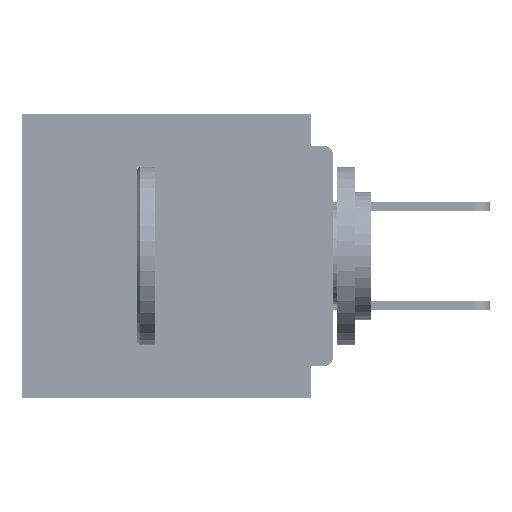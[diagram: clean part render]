
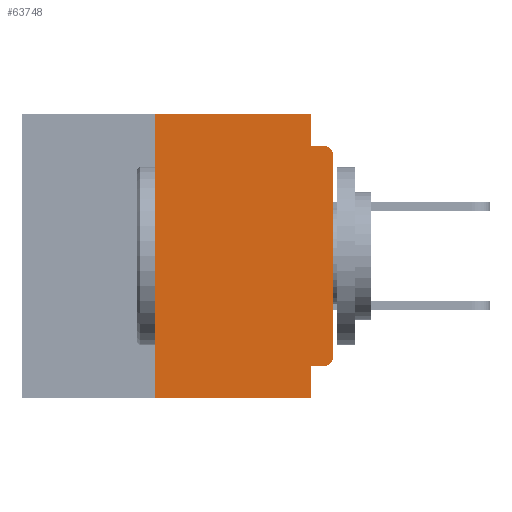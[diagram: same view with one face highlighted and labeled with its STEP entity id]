
A CAD part, left-side view. The second image highlights one B-rep face of the part: STEP entity #63748.
In plain terms, the highlighted planar face has unit normal (-1, 0, 0).
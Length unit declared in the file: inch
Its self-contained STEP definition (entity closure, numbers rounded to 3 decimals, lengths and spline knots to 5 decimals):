
#318 = VECTOR ( 'NONE', #19293, 39.37008 ) ;
#373 = AXIS2_PLACEMENT_3D ( 'NONE', #6621, #44049, #12014 ) ;
#502 = DIRECTION ( 'NONE',  ( 0., 0., -1. ) ) ;
#720 = DIRECTION ( 'NONE',  ( 0., -1., 0. ) ) ;
#1556 = LINE ( 'NONE', #37863, #56760 ) ;
#1593 = ORIENTED_EDGE ( 'NONE', *, *, #16591, .T. ) ;
#1703 = ORIENTED_EDGE ( 'NONE', *, *, #24254, .T. ) ;
#5988 = DIRECTION ( 'NONE',  ( 0., -1., 0. ) ) ;
#6621 = CARTESIAN_POINT ( 'NONE',  ( 0., 0.015, -0.06 ) ) ;
#6704 = CARTESIAN_POINT ( 'NONE',  ( 0., 0.25, -0.4 ) ) ;
#7061 = ORIENTED_EDGE ( 'NONE', *, *, #19541, .F. ) ;
#7080 = VERTEX_POINT ( 'NONE', #16770 ) ;
#7920 = CARTESIAN_POINT ( 'NONE',  ( 0., 0.015, -0.355 ) ) ;
#8393 = LINE ( 'NONE', #21086, #49386 ) ;
#10730 = CARTESIAN_POINT ( 'NONE',  ( 0., 0.031, -0.4 ) ) ;
#11118 = CARTESIAN_POINT ( 'NONE',  ( 0., 0.031, -0.045 ) ) ;
#11796 = EDGE_CURVE ( 'NONE', #28692, #24097, #1556, .T. ) ;
#12014 = DIRECTION ( 'NONE',  ( 0., 0., -1. ) ) ;
#14049 = ORIENTED_EDGE ( 'NONE', *, *, #39791, .F. ) ;
#15329 = CARTESIAN_POINT ( 'NONE',  ( 0., 0., -0.06 ) ) ;
#15574 = VECTOR ( 'NONE', #720, 39.37008 ) ;
#15869 = CIRCLE ( 'NONE', #67544, 0.015 ) ;
#16591 = EDGE_CURVE ( 'NONE', #50386, #50998, #15869, .T. ) ;
#16770 = CARTESIAN_POINT ( 'NONE',  ( 0., 0.25, 0. ) ) ;
#17990 = LINE ( 'NONE', #56745, #48069 ) ;
#19293 = DIRECTION ( 'NONE',  ( 0., -1., 0. ) ) ;
#19541 = EDGE_CURVE ( 'NONE', #57576, #57256, #17990, .T. ) ;
#20749 = LINE ( 'NONE', #10730, #59945 ) ;
#21086 = CARTESIAN_POINT ( 'NONE',  ( 0., 0., 0. ) ) ;
#22308 = VECTOR ( 'NONE', #65503, 39.37008 ) ;
#24097 = VERTEX_POINT ( 'NONE', #42910 ) ;
#24254 = EDGE_CURVE ( 'NONE', #61625, #25536, #49575, .T. ) ;
#25517 = LINE ( 'NONE', #40756, #318 ) ;
#25536 = VERTEX_POINT ( 'NONE', #34360 ) ;
#27920 = PLANE ( 'NONE',  #44784 ) ;
#28692 = VERTEX_POINT ( 'NONE', #41600 ) ;
#30058 = CARTESIAN_POINT ( 'NONE',  ( 0., 0.031, 0. ) ) ;
#30346 = VERTEX_POINT ( 'NONE', #67611 ) ;
#32231 = ORIENTED_EDGE ( 'NONE', *, *, #11796, .T. ) ;
#32623 = DIRECTION ( 'NONE',  ( -1., 0., 0. ) ) ;
#33319 = DIRECTION ( 'NONE',  ( 0., 0., -1. ) ) ;
#34360 = CARTESIAN_POINT ( 'NONE',  ( 0., 0.015, -0.045 ) ) ;
#35379 = EDGE_CURVE ( 'NONE', #50998, #61625, #8393, .T. ) ;
#35638 = FACE_OUTER_BOUND ( 'NONE', #60972, .T. ) ;
#36778 = EDGE_CURVE ( 'NONE', #50386, #30346, #43433, .T. ) ;
#37863 = CARTESIAN_POINT ( 'NONE',  ( 0., 0.437, -0.4 ) ) ;
#39791 = EDGE_CURVE ( 'NONE', #30346, #24097, #20749, .T. ) ;
#40417 = ORIENTED_EDGE ( 'NONE', *, *, #45718, .F. ) ;
#40422 = CARTESIAN_POINT ( 'NONE',  ( 0., 0., -0.355 ) ) ;
#40756 = CARTESIAN_POINT ( 'NONE',  ( 0., 0., -0.045 ) ) ;
#41351 = EDGE_CURVE ( 'NONE', #7080, #57576, #58167, .T. ) ;
#41600 = CARTESIAN_POINT ( 'NONE',  ( 0., 0.25, -0.4 ) ) ;
#42910 = CARTESIAN_POINT ( 'NONE',  ( 0., 0.031, -0.4 ) ) ;
#43433 = LINE ( 'NONE', #40422, #55933 ) ;
#43937 = ORIENTED_EDGE ( 'NONE', *, *, #35379, .T. ) ;
#44049 = DIRECTION ( 'NONE',  ( -1., 0., 0. ) ) ;
#44784 = AXIS2_PLACEMENT_3D ( 'NONE', #59848, #65178, #33319 ) ;
#44824 = EDGE_CURVE ( 'NONE', #28692, #7080, #64791, .T. ) ;
#45331 = ORIENTED_EDGE ( 'NONE', *, *, #41351, .F. ) ;
#45718 = EDGE_CURVE ( 'NONE', #57256, #25536, #25517, .T. ) ;
#47567 = ORIENTED_EDGE ( 'NONE', *, *, #44824, .F. ) ;
#48069 = VECTOR ( 'NONE', #51179, 39.37008 ) ;
#49386 = VECTOR ( 'NONE', #53065, 39.37008 ) ;
#49575 = CIRCLE ( 'NONE', #373, 0.015 ) ;
#50386 = VERTEX_POINT ( 'NONE', #7920 ) ;
#50998 = VERTEX_POINT ( 'NONE', #66387 ) ;
#51179 = DIRECTION ( 'NONE',  ( 0., 0., -1. ) ) ;
#53065 = DIRECTION ( 'NONE',  ( 0., 0., 1. ) ) ;
#53484 = DIRECTION ( 'NONE',  ( 0., 0., -1. ) ) ;
#55933 = VECTOR ( 'NONE', #66901, 39.37008 ) ;
#56745 = CARTESIAN_POINT ( 'NONE',  ( 0., 0.031, 0. ) ) ;
#56760 = VECTOR ( 'NONE', #5988, 39.37008 ) ;
#57256 = VERTEX_POINT ( 'NONE', #11118 ) ;
#57576 = VERTEX_POINT ( 'NONE', #30058 ) ;
#58167 = LINE ( 'NONE', #64713, #15574 ) ;
#59508 = ORIENTED_EDGE ( 'NONE', *, *, #36778, .F. ) ;
#59848 = CARTESIAN_POINT ( 'NONE',  ( 0., 0.437, 0. ) ) ;
#59945 = VECTOR ( 'NONE', #53484, 39.37008 ) ;
#60972 = EDGE_LOOP ( 'NONE', ( #43937, #1703, #40417, #7061, #45331, #47567, #32231, #14049, #59508, #1593 ) ) ;
#61625 = VERTEX_POINT ( 'NONE', #15329 ) ;
#63748 = ADVANCED_FACE ( 'NONE', ( #35638 ), #27920, .F. ) ;
#64490 = CARTESIAN_POINT ( 'NONE',  ( 0., 0.015, -0.34 ) ) ;
#64713 = CARTESIAN_POINT ( 'NONE',  ( 0., 0.437, 0. ) ) ;
#64791 = LINE ( 'NONE', #6704, #22308 ) ;
#65178 = DIRECTION ( 'NONE',  ( 1., 0., 0. ) ) ;
#65503 = DIRECTION ( 'NONE',  ( 0., 0., 1. ) ) ;
#66387 = CARTESIAN_POINT ( 'NONE',  ( 0., 0., -0.34 ) ) ;
#66901 = DIRECTION ( 'NONE',  ( 0., 1., 0. ) ) ;
#67544 = AXIS2_PLACEMENT_3D ( 'NONE', #64490, #32623, #502 ) ;
#67611 = CARTESIAN_POINT ( 'NONE',  ( 0., 0.031, -0.355 ) ) ;
